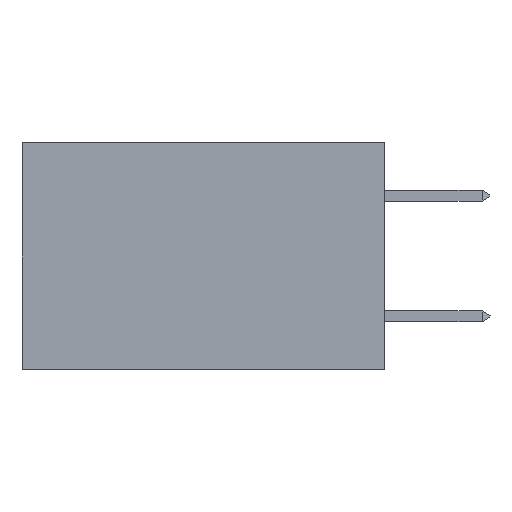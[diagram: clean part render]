
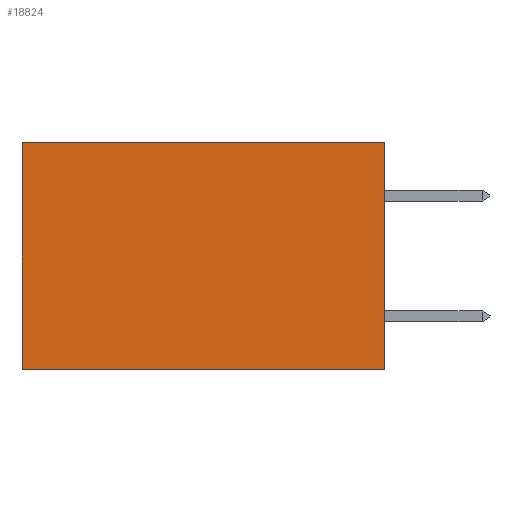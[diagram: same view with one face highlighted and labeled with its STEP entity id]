
A CAD part, left-side view. The second image highlights one B-rep face of the part: STEP entity #18824.
In plain terms, the highlighted planar face has unit normal (-1, 0, 0).
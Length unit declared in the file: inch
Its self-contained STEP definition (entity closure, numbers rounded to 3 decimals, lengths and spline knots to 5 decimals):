
#308 = VERTEX_POINT ( 'NONE', #14972 ) ;
#518 = CARTESIAN_POINT ( 'NONE',  ( 0.2875, 0.6, 0. ) ) ;
#1225 = PLANE ( 'NONE',  #9695 ) ;
#1303 = VECTOR ( 'NONE', #21270, 39.37008 ) ;
#1316 = EDGE_LOOP ( 'NONE', ( #19152, #21088, #13685, #15021 ) ) ;
#1828 = LINE ( 'NONE', #13030, #1303 ) ;
#1952 = VECTOR ( 'NONE', #11800, 39.37008 ) ;
#2954 = EDGE_CURVE ( 'NONE', #15053, #13830, #15425, .T. ) ;
#6788 = FACE_OUTER_BOUND ( 'NONE', #1316, .T. ) ;
#7919 = DIRECTION ( 'NONE',  ( 0., 0., -1. ) ) ;
#7994 = CARTESIAN_POINT ( 'NONE',  ( 0.2875, 0., -0.375 ) ) ;
#8019 = EDGE_CURVE ( 'NONE', #308, #20297, #1828, .T. ) ;
#9695 = AXIS2_PLACEMENT_3D ( 'NONE', #7994, #12971, #7919 ) ;
#10006 = CARTESIAN_POINT ( 'NONE',  ( 0.2875, 0., -0.375 ) ) ;
#10706 = CARTESIAN_POINT ( 'NONE',  ( 0.2875, 0., 0. ) ) ;
#10889 = CARTESIAN_POINT ( 'NONE',  ( 0.2875, 0.6, -0.375 ) ) ;
#11588 = DIRECTION ( 'NONE',  ( 0., 0., -1. ) ) ;
#11800 = DIRECTION ( 'NONE',  ( 0., 1., 0. ) ) ;
#12310 = DIRECTION ( 'NONE',  ( 0., 1., 0. ) ) ;
#12560 = VECTOR ( 'NONE', #11588, 39.37008 ) ;
#12971 = DIRECTION ( 'NONE',  ( 1., 0., 0. ) ) ;
#13030 = CARTESIAN_POINT ( 'NONE',  ( 0.2875, 0., -0.375 ) ) ;
#13685 = ORIENTED_EDGE ( 'NONE', *, *, #8019, .F. ) ;
#13830 = VERTEX_POINT ( 'NONE', #10889 ) ;
#14972 = CARTESIAN_POINT ( 'NONE',  ( 0.2875, 0., 0. ) ) ;
#15021 = ORIENTED_EDGE ( 'NONE', *, *, #21731, .T. ) ;
#15053 = VERTEX_POINT ( 'NONE', #518 ) ;
#15425 = LINE ( 'NONE', #19591, #12560 ) ;
#15440 = EDGE_CURVE ( 'NONE', #20297, #13830, #16646, .T. ) ;
#16646 = LINE ( 'NONE', #20184, #1952 ) ;
#17560 = LINE ( 'NONE', #10706, #19146 ) ;
#18824 = ADVANCED_FACE ( 'NONE', ( #6788 ), #1225, .F. ) ;
#19146 = VECTOR ( 'NONE', #12310, 39.37008 ) ;
#19152 = ORIENTED_EDGE ( 'NONE', *, *, #2954, .T. ) ;
#19591 = CARTESIAN_POINT ( 'NONE',  ( 0.2875, 0.6, -0.375 ) ) ;
#20184 = CARTESIAN_POINT ( 'NONE',  ( 0.2875, 0., -0.375 ) ) ;
#20297 = VERTEX_POINT ( 'NONE', #10006 ) ;
#21088 = ORIENTED_EDGE ( 'NONE', *, *, #15440, .F. ) ;
#21270 = DIRECTION ( 'NONE',  ( 0., 0., -1. ) ) ;
#21731 = EDGE_CURVE ( 'NONE', #308, #15053, #17560, .T. ) ;
